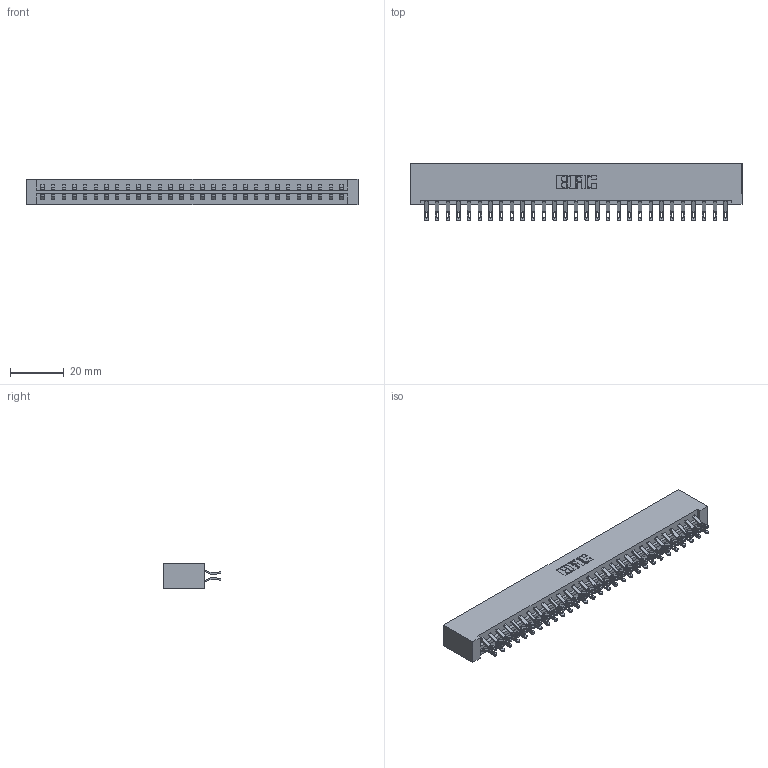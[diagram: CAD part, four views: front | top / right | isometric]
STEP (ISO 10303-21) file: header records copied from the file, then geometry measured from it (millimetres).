
FILE_DESCRIPTION (( 'STEP AP203' ), '1' );
FILE_NAME ('833-058-555-201.STEP', '2020-06-05T00:58:40', ( '' ), ( '' ), 'SwSTEP 2.0', 'SolidWorks 2020', '' );
FILE_SCHEMA (( 'CONFIG_CONTROL_DESIGN' ));
Length unit declared in the file: inch
Products named in the file (3): 833 Part_Lugless; 833-058-555-201; 345-292-001_555 Tail
Assembly tree (59 placements, depth 2):
  833-058-555-201
    833 Part_Lugless
    345-292-001_555 Tail  x58
Bounding box: 123.16 x 21.47 x 9.4 mm (x, y, z)
Volume: 13253.3 mm3; surface area: 16182.5 mm2
Topology: 59 solids, 59 shells, 3470 faces, 10901 edges, 7266 vertices
Faces by surface type: plane 2038, cylinder 1432
Entity records: 20387 total; most frequent: CARTESIAN_POINT 3428, ORIENTED_EDGE 3334, DIRECTION 2915, EDGE_CURVE 1667, VECTOR 1527, LINE 1527, VERTEX_POINT 1110, AXIS2_PLACEMENT_3D 694
